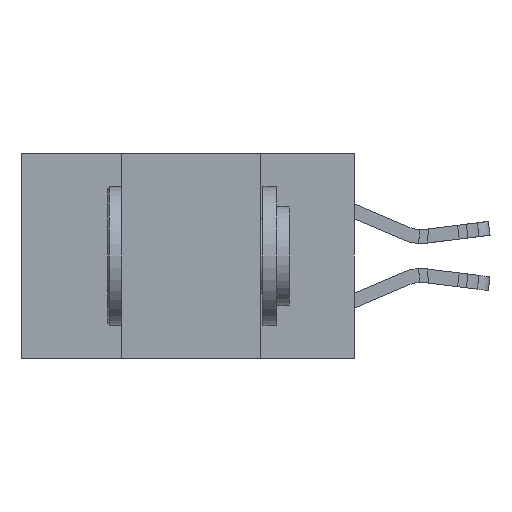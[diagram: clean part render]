
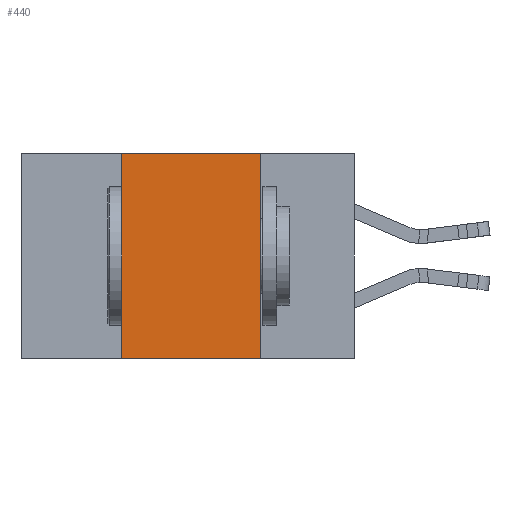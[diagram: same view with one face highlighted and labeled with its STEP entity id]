
A CAD part, left-side view. The second image highlights one B-rep face of the part: STEP entity #440.
In plain terms, the highlighted planar face has unit normal (-1, 0, 0).
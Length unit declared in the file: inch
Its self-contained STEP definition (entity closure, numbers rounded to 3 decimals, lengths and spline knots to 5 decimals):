
#440 = ADVANCED_FACE ( 'NONE', ( #2745 ), #26678, .F. ) ;
#603 = EDGE_LOOP ( 'NONE', ( #21766, #10865, #10801, #4839 ) ) ;
#1812 = LINE ( 'NONE', #19498, #13432 ) ;
#2361 = VECTOR ( 'NONE', #23800, 39.37008 ) ;
#2745 = FACE_OUTER_BOUND ( 'NONE', #603, .T. ) ;
#3395 = VERTEX_POINT ( 'NONE', #14989 ) ;
#4258 = CARTESIAN_POINT ( 'NONE',  ( 0., 0.6, -0.37 ) ) ;
#4449 = DIRECTION ( 'NONE',  ( 0., 0., -1. ) ) ;
#4839 = ORIENTED_EDGE ( 'NONE', *, *, #17850, .T. ) ;
#4863 = VECTOR ( 'NONE', #5754, 39.37008 ) ;
#5673 = DIRECTION ( 'NONE',  ( 0., 0., 1. ) ) ;
#5754 = DIRECTION ( 'NONE',  ( 0., -1., 0. ) ) ;
#6871 = DIRECTION ( 'NONE',  ( 1., 0., 0. ) ) ;
#8179 = CARTESIAN_POINT ( 'NONE',  ( 0., 0.17, 0. ) ) ;
#8941 = EDGE_CURVE ( 'NONE', #10689, #14363, #1812, .T. ) ;
#10497 = DIRECTION ( 'NONE',  ( 0., 0., -1. ) ) ;
#10689 = VERTEX_POINT ( 'NONE', #8179 ) ;
#10801 = ORIENTED_EDGE ( 'NONE', *, *, #13899, .F. ) ;
#10865 = ORIENTED_EDGE ( 'NONE', *, *, #24291, .F. ) ;
#13432 = VECTOR ( 'NONE', #10497, 39.37008 ) ;
#13899 = EDGE_CURVE ( 'NONE', #15412, #3395, #25216, .T. ) ;
#14060 = CARTESIAN_POINT ( 'NONE',  ( 0., 0.17, -0.37 ) ) ;
#14363 = VERTEX_POINT ( 'NONE', #14060 ) ;
#14989 = CARTESIAN_POINT ( 'NONE',  ( 0., 0.42, 0. ) ) ;
#15412 = VERTEX_POINT ( 'NONE', #16997 ) ;
#15846 = CARTESIAN_POINT ( 'NONE',  ( 0., 0.6, 0. ) ) ;
#16997 = CARTESIAN_POINT ( 'NONE',  ( 0., 0.42, -0.37 ) ) ;
#17850 = EDGE_CURVE ( 'NONE', #15412, #14363, #27805, .T. ) ;
#18296 = AXIS2_PLACEMENT_3D ( 'NONE', #15846, #6871, #4449 ) ;
#18753 = CARTESIAN_POINT ( 'NONE',  ( 0., 0.6, 0. ) ) ;
#19498 = CARTESIAN_POINT ( 'NONE',  ( 0., 0.17, -0.37 ) ) ;
#20506 = VECTOR ( 'NONE', #5673, 39.37008 ) ;
#21766 = ORIENTED_EDGE ( 'NONE', *, *, #8941, .F. ) ;
#23710 = LINE ( 'NONE', #18753, #4863 ) ;
#23800 = DIRECTION ( 'NONE',  ( 0., -1., 0. ) ) ;
#24291 = EDGE_CURVE ( 'NONE', #3395, #10689, #23710, .T. ) ;
#25216 = LINE ( 'NONE', #27496, #20506 ) ;
#26678 = PLANE ( 'NONE',  #18296 ) ;
#27496 = CARTESIAN_POINT ( 'NONE',  ( 0., 0.42, -0.37 ) ) ;
#27805 = LINE ( 'NONE', #4258, #2361 ) ;
